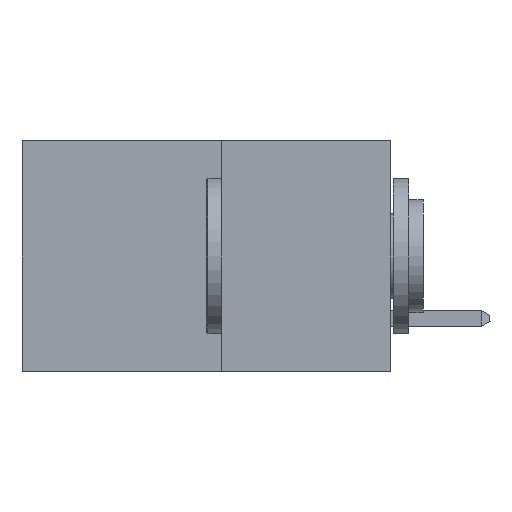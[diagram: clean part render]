
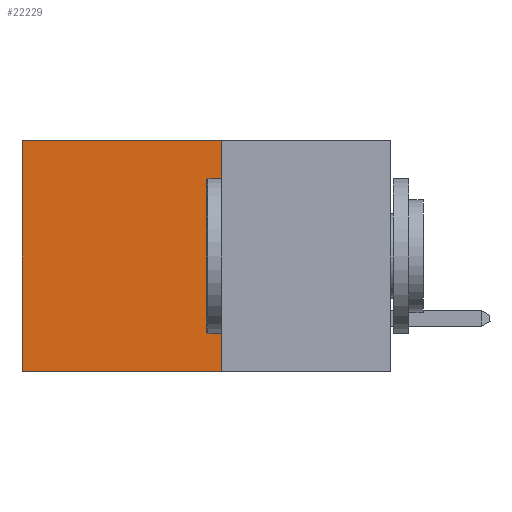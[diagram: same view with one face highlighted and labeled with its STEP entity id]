
A CAD part, left-side view. The second image highlights one B-rep face of the part: STEP entity #22229.
In plain terms, the highlighted planar face has unit normal (-1, 0, 0).
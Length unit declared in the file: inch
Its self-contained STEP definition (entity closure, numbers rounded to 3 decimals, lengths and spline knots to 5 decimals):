
#643 = EDGE_LOOP ( 'NONE', ( #1456, #21939, #18060, #21654 ) ) ;
#914 = CARTESIAN_POINT ( 'NONE',  ( 0.277, 0.27, -0.37 ) ) ;
#1319 = LINE ( 'NONE', #9455, #24881 ) ;
#1456 = ORIENTED_EDGE ( 'NONE', *, *, #8998, .T. ) ;
#3861 = CARTESIAN_POINT ( 'NONE',  ( 0.277, 0.27, 0. ) ) ;
#4050 = DIRECTION ( 'NONE',  ( 0., 1., 0. ) ) ;
#5321 = EDGE_CURVE ( 'NONE', #24440, #17959, #8982, .T. ) ;
#8170 = FACE_OUTER_BOUND ( 'NONE', #643, .T. ) ;
#8564 = LINE ( 'NONE', #17711, #20729 ) ;
#8743 = DIRECTION ( 'NONE',  ( 0., 0., -1. ) ) ;
#8982 = LINE ( 'NONE', #26124, #14357 ) ;
#8998 = EDGE_CURVE ( 'NONE', #17959, #18417, #1319, .T. ) ;
#9455 = CARTESIAN_POINT ( 'NONE',  ( 0.277, 0.59, -0.37 ) ) ;
#12309 = CARTESIAN_POINT ( 'NONE',  ( 0.277, 0.27, -0.37 ) ) ;
#14064 = DIRECTION ( 'NONE',  ( 0., 0., -1. ) ) ;
#14357 = VECTOR ( 'NONE', #14743, 39.37008 ) ;
#14743 = DIRECTION ( 'NONE',  ( 0., 1., 0. ) ) ;
#17399 = VECTOR ( 'NONE', #21531, 39.37008 ) ;
#17711 = CARTESIAN_POINT ( 'NONE',  ( 0.277, 0.27, -0.37 ) ) ;
#17843 = PLANE ( 'NONE',  #19518 ) ;
#17959 = VERTEX_POINT ( 'NONE', #21583 ) ;
#18060 = ORIENTED_EDGE ( 'NONE', *, *, #19137, .F. ) ;
#18118 = LINE ( 'NONE', #12309, #17399 ) ;
#18417 = VERTEX_POINT ( 'NONE', #25227 ) ;
#19137 = EDGE_CURVE ( 'NONE', #24440, #29103, #18118, .T. ) ;
#19518 = AXIS2_PLACEMENT_3D ( 'NONE', #20154, #22465, #8743 ) ;
#20154 = CARTESIAN_POINT ( 'NONE',  ( 0.277, 0.27, -0.37 ) ) ;
#20729 = VECTOR ( 'NONE', #4050, 39.37008 ) ;
#20850 = EDGE_CURVE ( 'NONE', #29103, #18417, #8564, .T. ) ;
#21531 = DIRECTION ( 'NONE',  ( 0., 0., -1. ) ) ;
#21583 = CARTESIAN_POINT ( 'NONE',  ( 0.277, 0.59, 0. ) ) ;
#21654 = ORIENTED_EDGE ( 'NONE', *, *, #5321, .T. ) ;
#21939 = ORIENTED_EDGE ( 'NONE', *, *, #20850, .F. ) ;
#22229 = ADVANCED_FACE ( 'NONE', ( #8170 ), #17843, .F. ) ;
#22465 = DIRECTION ( 'NONE',  ( 1., 0., 0. ) ) ;
#24440 = VERTEX_POINT ( 'NONE', #3861 ) ;
#24881 = VECTOR ( 'NONE', #14064, 39.37008 ) ;
#25227 = CARTESIAN_POINT ( 'NONE',  ( 0.277, 0.59, -0.37 ) ) ;
#26124 = CARTESIAN_POINT ( 'NONE',  ( 0.277, 0.27, 0. ) ) ;
#29103 = VERTEX_POINT ( 'NONE', #914 ) ;
